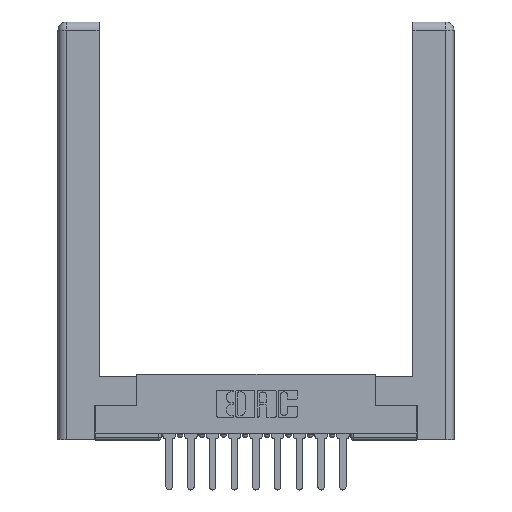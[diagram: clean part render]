
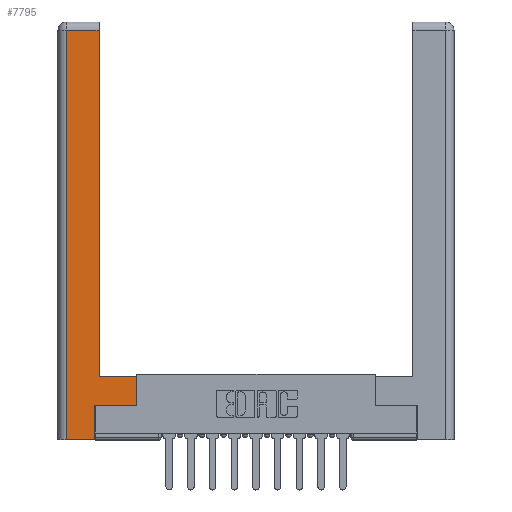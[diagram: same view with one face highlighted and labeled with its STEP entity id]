
A CAD part, top view. The second image highlights one B-rep face of the part: STEP entity #7795.
In plain terms, the highlighted planar face has unit normal (0, 0, 1).
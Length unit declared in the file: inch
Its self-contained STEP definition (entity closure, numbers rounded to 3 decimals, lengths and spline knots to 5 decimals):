
#299 = CARTESIAN_POINT ( 'NONE',  ( 0.0615, 0., 0. ) ) ;
#391 = DIRECTION ( 'NONE',  ( -1., 0., 0. ) ) ;
#490 = VECTOR ( 'NONE', #6391, 39.37008 ) ;
#495 = CARTESIAN_POINT ( 'NONE',  ( 0.295, 0.45, 0. ) ) ;
#624 = LINE ( 'NONE', #12574, #9329 ) ;
#1085 = EDGE_CURVE ( 'NONE', #12408, #9749, #1553, .T. ) ;
#1113 = VERTEX_POINT ( 'NONE', #10965 ) ;
#1219 = CARTESIAN_POINT ( 'NONE',  ( 0.265, 0.245, 0. ) ) ;
#1539 = CARTESIAN_POINT ( 'NONE',  ( 0.295, 3., 0. ) ) ;
#1553 = LINE ( 'NONE', #1539, #490 ) ;
#1640 = ORIENTED_EDGE ( 'NONE', *, *, #5948, .T. ) ;
#1919 = DIRECTION ( 'NONE',  ( 1., 0., 0. ) ) ;
#2141 = CARTESIAN_POINT ( 'NONE',  ( 0.565, 0.45, 0. ) ) ;
#2376 = EDGE_CURVE ( 'NONE', #6501, #3012, #624, .T. ) ;
#2417 = VECTOR ( 'NONE', #4714, 39.37008 ) ;
#2742 = CARTESIAN_POINT ( 'NONE',  ( 0.295, 0.45, 0. ) ) ;
#2953 = ORIENTED_EDGE ( 'NONE', *, *, #7693, .T. ) ;
#3012 = VERTEX_POINT ( 'NONE', #9369 ) ;
#3152 = LINE ( 'NONE', #14275, #5448 ) ;
#3171 = ORIENTED_EDGE ( 'NONE', *, *, #2376, .T. ) ;
#3479 = LINE ( 'NONE', #495, #2417 ) ;
#3650 = VERTEX_POINT ( 'NONE', #2141 ) ;
#3709 = CARTESIAN_POINT ( 'NONE',  ( 0.265, 0.245, 0. ) ) ;
#3792 = VECTOR ( 'NONE', #5866, 39.37008 ) ;
#3793 = ORIENTED_EDGE ( 'NONE', *, *, #10149, .T. ) ;
#4129 = FACE_OUTER_BOUND ( 'NONE', #6071, .T. ) ;
#4714 = DIRECTION ( 'NONE',  ( -1., 0., 0. ) ) ;
#4776 = CARTESIAN_POINT ( 'NONE',  ( 0.0615, 0., 0. ) ) ;
#4838 = VECTOR ( 'NONE', #391, 39.37008 ) ;
#5448 = VECTOR ( 'NONE', #1919, 39.37008 ) ;
#5501 = DIRECTION ( 'NONE',  ( 0., 0., -1. ) ) ;
#5866 = DIRECTION ( 'NONE',  ( 0., -1., 0. ) ) ;
#5948 = EDGE_CURVE ( 'NONE', #3012, #10843, #8859, .T. ) ;
#5990 = CARTESIAN_POINT ( 'NONE',  ( 0.565, 0.245, 0. ) ) ;
#6071 = EDGE_LOOP ( 'NONE', ( #13105, #9123, #2953, #3171, #1640, #6751, #3793, #12787 ) ) ;
#6391 = DIRECTION ( 'NONE',  ( 0., 1., 0. ) ) ;
#6501 = VERTEX_POINT ( 'NONE', #299 ) ;
#6507 = VERTEX_POINT ( 'NONE', #5990 ) ;
#6526 = CARTESIAN_POINT ( 'NONE',  ( 0.565, 0.45, 0. ) ) ;
#6751 = ORIENTED_EDGE ( 'NONE', *, *, #7361, .T. ) ;
#7187 = DIRECTION ( 'NONE',  ( 0., 1., 0. ) ) ;
#7361 = EDGE_CURVE ( 'NONE', #10843, #6507, #3152, .T. ) ;
#7693 = EDGE_CURVE ( 'NONE', #1113, #6501, #9670, .T. ) ;
#7780 = DIRECTION ( 'NONE',  ( 0., 1., 0. ) ) ;
#7795 = ADVANCED_FACE ( 'NONE', ( #4129 ), #13570, .F. ) ;
#8372 = EDGE_CURVE ( 'NONE', #9749, #1113, #13211, .T. ) ;
#8859 = LINE ( 'NONE', #3709, #13132 ) ;
#9123 = ORIENTED_EDGE ( 'NONE', *, *, #8372, .T. ) ;
#9329 = VECTOR ( 'NONE', #10215, 39.37008 ) ;
#9369 = CARTESIAN_POINT ( 'NONE',  ( 0.265, 0., 0. ) ) ;
#9670 = LINE ( 'NONE', #4776, #3792 ) ;
#9749 = VERTEX_POINT ( 'NONE', #13815 ) ;
#10149 = EDGE_CURVE ( 'NONE', #6507, #3650, #10814, .T. ) ;
#10215 = DIRECTION ( 'NONE',  ( 1., 0., 0. ) ) ;
#10814 = LINE ( 'NONE', #6526, #11713 ) ;
#10843 = VERTEX_POINT ( 'NONE', #1219 ) ;
#10965 = CARTESIAN_POINT ( 'NONE',  ( 0.0615, 2.94, 0. ) ) ;
#11713 = VECTOR ( 'NONE', #7780, 39.37008 ) ;
#11722 = CARTESIAN_POINT ( 'NONE',  ( 0.0615, 2.94, 0. ) ) ;
#12335 = CARTESIAN_POINT ( 'NONE',  ( 0., 0., 0. ) ) ;
#12408 = VERTEX_POINT ( 'NONE', #2742 ) ;
#12574 = CARTESIAN_POINT ( 'NONE',  ( 0.265, 0., 0. ) ) ;
#12787 = ORIENTED_EDGE ( 'NONE', *, *, #12999, .T. ) ;
#12999 = EDGE_CURVE ( 'NONE', #3650, #12408, #3479, .T. ) ;
#13105 = ORIENTED_EDGE ( 'NONE', *, *, #1085, .T. ) ;
#13132 = VECTOR ( 'NONE', #7187, 39.37008 ) ;
#13135 = AXIS2_PLACEMENT_3D ( 'NONE', #12335, #5501, #13417 ) ;
#13211 = LINE ( 'NONE', #11722, #4838 ) ;
#13417 = DIRECTION ( 'NONE',  ( -1., 0., 0. ) ) ;
#13570 = PLANE ( 'NONE',  #13135 ) ;
#13815 = CARTESIAN_POINT ( 'NONE',  ( 0.295, 2.94, 0. ) ) ;
#14275 = CARTESIAN_POINT ( 'NONE',  ( 0.565, 0.245, 0. ) ) ;
